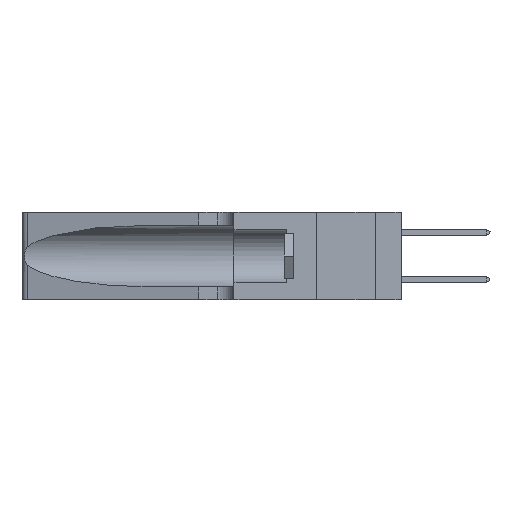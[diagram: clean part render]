
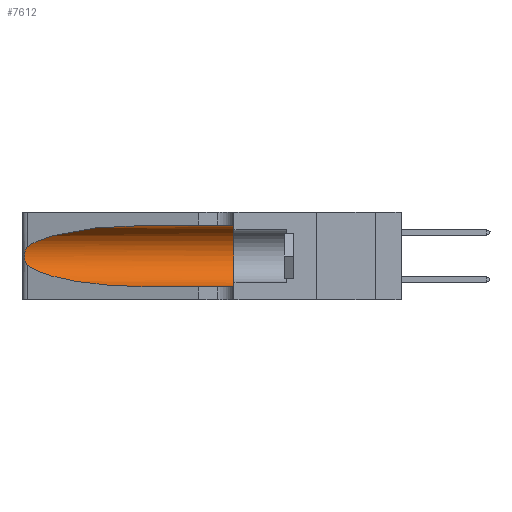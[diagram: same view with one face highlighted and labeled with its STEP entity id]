
A CAD part, left-side view. The second image highlights one B-rep face of the part: STEP entity #7612.
In plain terms, the highlighted cylindrical face has radius 3.308 mm (diameter 6.617 mm), a partial arc.
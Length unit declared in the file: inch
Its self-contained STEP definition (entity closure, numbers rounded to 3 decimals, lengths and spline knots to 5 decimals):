
#496 = CARTESIAN_POINT ( 'NONE',  ( 0.26018, 1.23835, 0.19895 ) ) ;
#600 = CARTESIAN_POINT ( 'NONE',  ( 0.18966, 0.96281, 0.31525 ) ) ;
#761 = LINE ( 'NONE', #30862, #17816 ) ;
#1025 = CARTESIAN_POINT ( 'NONE',  ( 0.25639, 1.23186, 0.15144 ) ) ;
#3587 = CARTESIAN_POINT ( 'NONE',  ( 0.25487, 1.22718, 0.22369 ) ) ;
#3713 = VERTEX_POINT ( 'NONE', #5534 ) ;
#5045 = EDGE_LOOP ( 'NONE', ( #18541, #17894, #8030, #37037, #36735, #26829 ) ) ;
#5534 = CARTESIAN_POINT ( 'NONE',  ( 0.25487, 1.22718, 0.22369 ) ) ;
#6693 = B_SPLINE_CURVE_WITH_KNOTS ( 'NONE', 3,
 ( #3587, #12485, #32644, #9246, #35836, #496, #26906, #29966, #21292, #29715, #9382, #1025, #12356, #12241 ),
 .UNSPECIFIED., .F., .F.,
 ( 4, 2, 2, 2, 2, 2, 4 ),
 ( 0., 0.00027, 0.00053, 0.00107, 0.0016, 0.00187, 0.00214 ),
 .UNSPECIFIED. ) ;
#7612 = ADVANCED_FACE ( 'NONE', ( #23808 ), #26108, .F. ) ;
#8030 = ORIENTED_EDGE ( 'NONE', *, *, #18453, .T. ) ;
#9110 = CARTESIAN_POINT ( 'NONE',  ( 0.1305, 0.35, 0.05475 ) ) ;
#9246 = CARTESIAN_POINT ( 'NONE',  ( 0.25787, 1.23484, 0.2124 ) ) ;
#9382 = CARTESIAN_POINT ( 'NONE',  ( 0.25789, 1.23486, 0.15765 ) ) ;
#9503 = EDGE_CURVE ( 'NONE', #21325, #3713, #21996, .T. ) ;
#9919 = CARTESIAN_POINT ( 'NONE',  ( 0.2373, 1.15595, 0.08982 ) ) ;
#10025 = EDGE_CURVE ( 'NONE', #23516, #23322, #36412, .T. ) ;
#10750 =( BOUNDED_CURVE ( )  B_SPLINE_CURVE ( 3, ( #24236, #9919, #15730, #13288 ),
 .UNSPECIFIED., .F., .F. ) 
 B_SPLINE_CURVE_WITH_KNOTS ( ( 4, 4 ),
 ( 3.44316, 4.71239 ),
 .UNSPECIFIED. ) 
 CURVE ( )  GEOMETRIC_REPRESENTATION_ITEM ( )  RATIONAL_B_SPLINE_CURVE ( ( 1., 0.87, 0.87, 1. ) ) 
 REPRESENTATION_ITEM ( '' )  );
#11236 = DIRECTION ( 'NONE',  ( 0., 1., 0. ) ) ;
#12241 = CARTESIAN_POINT ( 'NONE',  ( 0.25487, 1.22718, 0.14631 ) ) ;
#12356 = CARTESIAN_POINT ( 'NONE',  ( 0.25555, 1.22993, 0.14849 ) ) ;
#12485 = CARTESIAN_POINT ( 'NONE',  ( 0.25555, 1.22994, 0.2215 ) ) ;
#13288 = CARTESIAN_POINT ( 'NONE',  ( 0.1305, 0.72297, 0.05475 ) ) ;
#14440 = EDGE_CURVE ( 'NONE', #3713, #17215, #6693, .T. ) ;
#15011 = CARTESIAN_POINT ( 'NONE',  ( 0.2373, 1.15595, 0.28018 ) ) ;
#15730 = CARTESIAN_POINT ( 'NONE',  ( 0.18966, 0.96281, 0.05475 ) ) ;
#16403 = VECTOR ( 'NONE', #36529, 39.37008 ) ;
#16453 = CARTESIAN_POINT ( 'NONE',  ( 0.25487, 1.22718, 0.14631 ) ) ;
#17215 = VERTEX_POINT ( 'NONE', #16453 ) ;
#17816 = VECTOR ( 'NONE', #22325, 39.37008 ) ;
#17894 = ORIENTED_EDGE ( 'NONE', *, *, #14440, .T. ) ;
#18453 = EDGE_CURVE ( 'NONE', #17215, #22118, #10750, .T. ) ;
#18541 = ORIENTED_EDGE ( 'NONE', *, *, #9503, .T. ) ;
#18571 = DIRECTION ( 'NONE',  ( 0., -1., 0. ) ) ;
#18590 = EDGE_CURVE ( 'NONE', #21325, #23516, #761, .T. ) ;
#19223 = CARTESIAN_POINT ( 'NONE',  ( 0.1305, 0.35, 0.31525 ) ) ;
#21263 = CARTESIAN_POINT ( 'NONE',  ( 0.1305, 0.72297, 0.31525 ) ) ;
#21292 = CARTESIAN_POINT ( 'NONE',  ( 0.26017, 1.23833, 0.17102 ) ) ;
#21325 = VERTEX_POINT ( 'NONE', #21263 ) ;
#21996 =( BOUNDED_CURVE ( )  B_SPLINE_CURVE ( 3, ( #28895, #600, #15011, #23422 ),
 .UNSPECIFIED., .F., .F. ) 
 B_SPLINE_CURVE_WITH_KNOTS ( ( 4, 4 ),
 ( 1.5708, 2.84003 ),
 .UNSPECIFIED. ) 
 CURVE ( )  GEOMETRIC_REPRESENTATION_ITEM ( )  RATIONAL_B_SPLINE_CURVE ( ( 1., 0.87, 0.87, 1. ) ) 
 REPRESENTATION_ITEM ( '' )  );
#22118 = VERTEX_POINT ( 'NONE', #35763 ) ;
#22325 = DIRECTION ( 'NONE',  ( 0., -1., 0. ) ) ;
#23322 = VERTEX_POINT ( 'NONE', #9110 ) ;
#23422 = CARTESIAN_POINT ( 'NONE',  ( 0.25487, 1.22718, 0.22369 ) ) ;
#23516 = VERTEX_POINT ( 'NONE', #19223 ) ;
#23808 = FACE_OUTER_BOUND ( 'NONE', #5045, .T. ) ;
#24236 = CARTESIAN_POINT ( 'NONE',  ( 0.25487, 1.22718, 0.14631 ) ) ;
#24646 = CARTESIAN_POINT ( 'NONE',  ( 0.1305, 1.61858, 0.05475 ) ) ;
#24772 = DIRECTION ( 'NONE',  ( 0., 0., -1. ) ) ;
#26108 = CYLINDRICAL_SURFACE ( 'NONE', #27077, 0.13025 ) ;
#26631 = AXIS2_PLACEMENT_3D ( 'NONE', #34600, #11236, #37532 ) ;
#26829 = ORIENTED_EDGE ( 'NONE', *, *, #18590, .F. ) ;
#26906 = CARTESIAN_POINT ( 'NONE',  ( 0.26075, 1.23896, 0.19203 ) ) ;
#27077 = AXIS2_PLACEMENT_3D ( 'NONE', #32950, #18571, #24772 ) ;
#28624 = EDGE_CURVE ( 'NONE', #22118, #23322, #36922, .T. ) ;
#28895 = CARTESIAN_POINT ( 'NONE',  ( 0.1305, 0.72297, 0.31525 ) ) ;
#29715 = CARTESIAN_POINT ( 'NONE',  ( 0.25856, 1.23593, 0.16098 ) ) ;
#29966 = CARTESIAN_POINT ( 'NONE',  ( 0.26075, 1.23896, 0.178 ) ) ;
#30862 = CARTESIAN_POINT ( 'NONE',  ( 0.1305, 1.61858, 0.31525 ) ) ;
#32644 = CARTESIAN_POINT ( 'NONE',  ( 0.25639, 1.23184, 0.21858 ) ) ;
#32950 = CARTESIAN_POINT ( 'NONE',  ( 0.1305, 1.61858, 0.185 ) ) ;
#34600 = CARTESIAN_POINT ( 'NONE',  ( 0.1305, 0.35, 0.185 ) ) ;
#35763 = CARTESIAN_POINT ( 'NONE',  ( 0.1305, 0.72297, 0.05475 ) ) ;
#35836 = CARTESIAN_POINT ( 'NONE',  ( 0.25854, 1.2359, 0.20912 ) ) ;
#36412 = CIRCLE ( 'NONE', #26631, 0.13025 ) ;
#36529 = DIRECTION ( 'NONE',  ( 0., -1., 0. ) ) ;
#36735 = ORIENTED_EDGE ( 'NONE', *, *, #10025, .F. ) ;
#36922 = LINE ( 'NONE', #24646, #16403 ) ;
#37037 = ORIENTED_EDGE ( 'NONE', *, *, #28624, .T. ) ;
#37532 = DIRECTION ( 'NONE',  ( 0., 0., 1. ) ) ;
